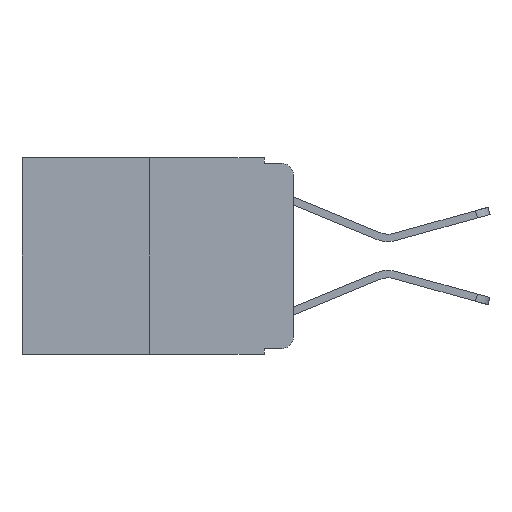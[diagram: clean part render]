
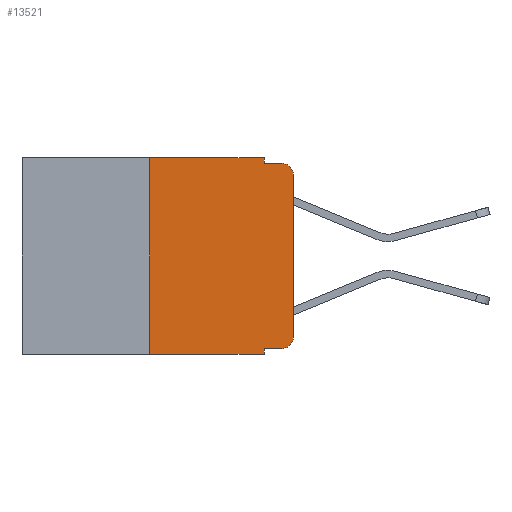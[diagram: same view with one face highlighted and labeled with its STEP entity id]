
A CAD part, left-side view. The second image highlights one B-rep face of the part: STEP entity #13521.
In plain terms, the highlighted planar face has unit normal (-1, 0, 0).
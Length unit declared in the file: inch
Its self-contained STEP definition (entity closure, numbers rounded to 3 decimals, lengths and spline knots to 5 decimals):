
#110 = LINE ( 'NONE', #3429, #2936 ) ;
#368 = ORIENTED_EDGE ( 'NONE', *, *, #4995, .F. ) ;
#438 = CARTESIAN_POINT ( 'NONE',  ( 0., 0.02, -0.01 ) ) ;
#1130 = DIRECTION ( 'NONE',  ( 1., 0., 0. ) ) ;
#1286 = DIRECTION ( 'NONE',  ( 0., -1., 0. ) ) ;
#1331 = CARTESIAN_POINT ( 'NONE',  ( 0., 0.25, 0. ) ) ;
#1624 = LINE ( 'NONE', #7325, #12029 ) ;
#1817 = EDGE_CURVE ( 'NONE', #6759, #10815, #12380, .T. ) ;
#2229 = CARTESIAN_POINT ( 'NONE',  ( 0., 0.051, 0. ) ) ;
#2307 = AXIS2_PLACEMENT_3D ( 'NONE', #8131, #14770, #14525 ) ;
#2564 = LINE ( 'NONE', #4505, #3308 ) ;
#2785 = LINE ( 'NONE', #6163, #14493 ) ;
#2835 = VECTOR ( 'NONE', #10592, 39.37008 ) ;
#2888 = LINE ( 'NONE', #11258, #6011 ) ;
#2936 = VECTOR ( 'NONE', #11427, 39.37008 ) ;
#3181 = ORIENTED_EDGE ( 'NONE', *, *, #1817, .T. ) ;
#3307 = CARTESIAN_POINT ( 'NONE',  ( 0., 0.473, 0. ) ) ;
#3308 = VECTOR ( 'NONE', #11332, 39.37008 ) ;
#3429 = CARTESIAN_POINT ( 'NONE',  ( 0., 0.051, 0. ) ) ;
#3554 = ORIENTED_EDGE ( 'NONE', *, *, #8820, .F. ) ;
#3809 = VERTEX_POINT ( 'NONE', #2229 ) ;
#3924 = ORIENTED_EDGE ( 'NONE', *, *, #5294, .F. ) ;
#3979 = AXIS2_PLACEMENT_3D ( 'NONE', #10352, #1130, #9279 ) ;
#4098 = EDGE_CURVE ( 'NONE', #12552, #4931, #9901, .T. ) ;
#4297 = ORIENTED_EDGE ( 'NONE', *, *, #12745, .T. ) ;
#4420 = DIRECTION ( 'NONE',  ( 0., 0., 1. ) ) ;
#4505 = CARTESIAN_POINT ( 'NONE',  ( 0., 0.051, 0. ) ) ;
#4709 = DIRECTION ( 'NONE',  ( 0., 0., -1. ) ) ;
#4931 = VERTEX_POINT ( 'NONE', #10247 ) ;
#4995 = EDGE_CURVE ( 'NONE', #9249, #10815, #9876, .T. ) ;
#5294 = EDGE_CURVE ( 'NONE', #11286, #3809, #9005, .T. ) ;
#5834 = CARTESIAN_POINT ( 'NONE',  ( 0., 0.051, -0.343 ) ) ;
#6011 = VECTOR ( 'NONE', #4420, 39.37008 ) ;
#6163 = CARTESIAN_POINT ( 'NONE',  ( 0., 0.473, -0.343 ) ) ;
#6759 = VERTEX_POINT ( 'NONE', #11044 ) ;
#6770 = DIRECTION ( 'NONE',  ( 0., -1., 0. ) ) ;
#7018 = ORIENTED_EDGE ( 'NONE', *, *, #14746, .F. ) ;
#7325 = CARTESIAN_POINT ( 'NONE',  ( 0., 0., 0. ) ) ;
#7329 = DIRECTION ( 'NONE',  ( 0., -1., 0. ) ) ;
#7347 = LINE ( 'NONE', #10167, #10339 ) ;
#7586 = VECTOR ( 'NONE', #1286, 39.37008 ) ;
#8131 = CARTESIAN_POINT ( 'NONE',  ( 0., 0.02, -0.313 ) ) ;
#8529 = CARTESIAN_POINT ( 'NONE',  ( 0., 0.25, -0.343 ) ) ;
#8820 = EDGE_CURVE ( 'NONE', #3809, #9249, #2564, .T. ) ;
#8821 = DIRECTION ( 'NONE',  ( -1., 0., 0. ) ) ;
#9005 = LINE ( 'NONE', #3307, #2835 ) ;
#9008 = CARTESIAN_POINT ( 'NONE',  ( 0., 0.02, -0.03 ) ) ;
#9031 = VERTEX_POINT ( 'NONE', #8529 ) ;
#9104 = CARTESIAN_POINT ( 'NONE',  ( 0., 0.051, -0.333 ) ) ;
#9249 = VERTEX_POINT ( 'NONE', #14486 ) ;
#9279 = DIRECTION ( 'NONE',  ( 0., 0., -1. ) ) ;
#9876 = LINE ( 'NONE', #14819, #7586 ) ;
#9901 = CIRCLE ( 'NONE', #2307, 0.02 ) ;
#10010 = ORIENTED_EDGE ( 'NONE', *, *, #12443, .T. ) ;
#10167 = CARTESIAN_POINT ( 'NONE',  ( 0., 0.051, -0.333 ) ) ;
#10247 = CARTESIAN_POINT ( 'NONE',  ( 0., 0., -0.313 ) ) ;
#10339 = VECTOR ( 'NONE', #6770, 39.37008 ) ;
#10352 = CARTESIAN_POINT ( 'NONE',  ( 0., 0.473, 0. ) ) ;
#10592 = DIRECTION ( 'NONE',  ( 0., -1., 0. ) ) ;
#10815 = VERTEX_POINT ( 'NONE', #438 ) ;
#11044 = CARTESIAN_POINT ( 'NONE',  ( 0., 0., -0.03 ) ) ;
#11258 = CARTESIAN_POINT ( 'NONE',  ( 0., 0.25, 0. ) ) ;
#11286 = VERTEX_POINT ( 'NONE', #1331 ) ;
#11332 = DIRECTION ( 'NONE',  ( 0., 0., -1. ) ) ;
#11427 = DIRECTION ( 'NONE',  ( 0., 0., -1. ) ) ;
#12029 = VECTOR ( 'NONE', #12847, 39.37008 ) ;
#12380 = CIRCLE ( 'NONE', #14109, 0.02 ) ;
#12443 = EDGE_CURVE ( 'NONE', #9031, #13519, #2785, .T. ) ;
#12552 = VERTEX_POINT ( 'NONE', #13092 ) ;
#12745 = EDGE_CURVE ( 'NONE', #12770, #12552, #7347, .T. ) ;
#12770 = VERTEX_POINT ( 'NONE', #9104 ) ;
#12847 = DIRECTION ( 'NONE',  ( 0., 0., 1. ) ) ;
#12973 = ORIENTED_EDGE ( 'NONE', *, *, #13483, .F. ) ;
#13092 = CARTESIAN_POINT ( 'NONE',  ( 0., 0.02, -0.333 ) ) ;
#13265 = EDGE_LOOP ( 'NONE', ( #14591, #3181, #368, #3554, #3924, #7018, #10010, #12973, #4297, #13324 ) ) ;
#13324 = ORIENTED_EDGE ( 'NONE', *, *, #4098, .T. ) ;
#13483 = EDGE_CURVE ( 'NONE', #12770, #13519, #110, .T. ) ;
#13519 = VERTEX_POINT ( 'NONE', #5834 ) ;
#13521 = ADVANCED_FACE ( 'NONE', ( #14282 ), #14776, .F. ) ;
#14109 = AXIS2_PLACEMENT_3D ( 'NONE', #9008, #8821, #4709 ) ;
#14282 = FACE_OUTER_BOUND ( 'NONE', #13265, .T. ) ;
#14288 = EDGE_CURVE ( 'NONE', #4931, #6759, #1624, .T. ) ;
#14486 = CARTESIAN_POINT ( 'NONE',  ( 0., 0.051, -0.01 ) ) ;
#14493 = VECTOR ( 'NONE', #7329, 39.37008 ) ;
#14525 = DIRECTION ( 'NONE',  ( 0., 0., -1. ) ) ;
#14591 = ORIENTED_EDGE ( 'NONE', *, *, #14288, .T. ) ;
#14746 = EDGE_CURVE ( 'NONE', #9031, #11286, #2888, .T. ) ;
#14770 = DIRECTION ( 'NONE',  ( -1., 0., 0. ) ) ;
#14776 = PLANE ( 'NONE',  #3979 ) ;
#14819 = CARTESIAN_POINT ( 'NONE',  ( 0., 0.051, -0.01 ) ) ;
